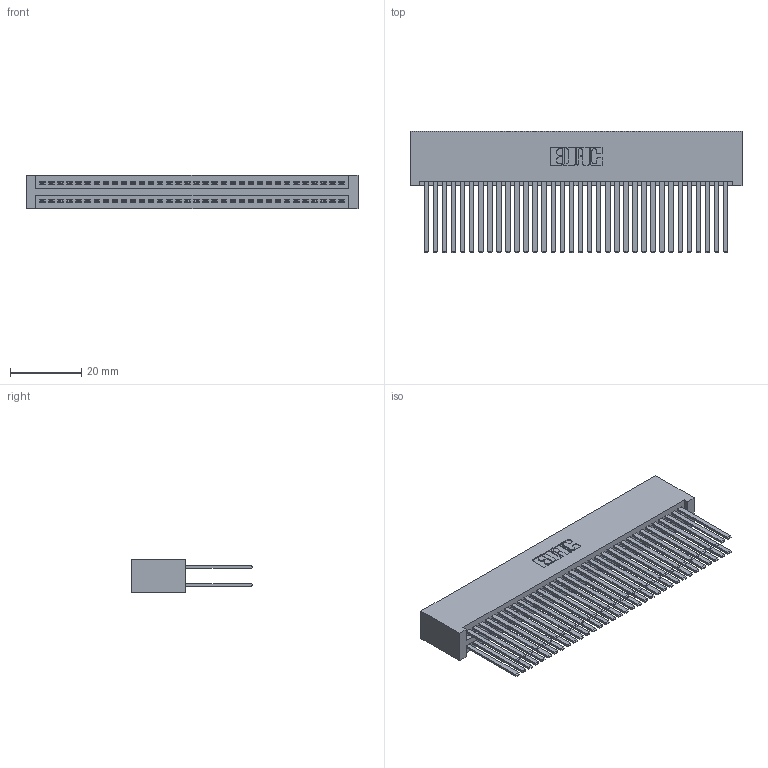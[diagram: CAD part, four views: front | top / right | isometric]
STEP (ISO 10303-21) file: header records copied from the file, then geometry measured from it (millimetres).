
FILE_DESCRIPTION (( 'STEP AP203' ), '1' );
FILE_NAME ('395-068-544-201.STEP', '2018-11-25T17:41:14', ( '' ), ( '' ), 'SwSTEP 2.0', 'SolidWorks 2016', '' );
FILE_SCHEMA (( 'CONFIG_CONTROL_DESIGN' ));
Length unit declared in the file: inch
Products named in the file (3): 345 Part_No Mounting Lugs; 345-292-001_345-293-144; 395-068-544-201
Assembly tree (69 placements, depth 2):
  395-068-544-201
    345 Part_No Mounting Lugs
    345-292-001_345-293-144  x68
Bounding box: 92.96 x 33.96 x 9.4 mm (x, y, z)
Volume: 10525.5 mm3; surface area: 18500.6 mm2
Topology: 69 solids, 69 shells, 3110 faces, 9225 edges, 6058 vertices
Faces by surface type: plane 2048, cylinder 1062
Entity records: 27293 total; most frequent: CARTESIAN_POINT 4580, ORIENTED_EDGE 4514, DIRECTION 4041, EDGE_CURVE 2257, VECTOR 2001, LINE 2001, VERTEX_POINT 1502, AXIS2_PLACEMENT_3D 1020
